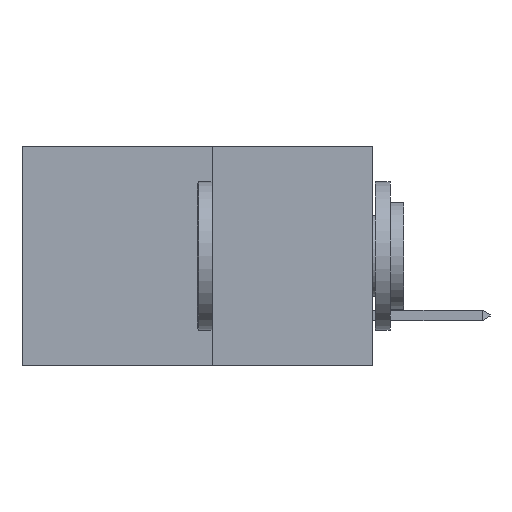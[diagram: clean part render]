
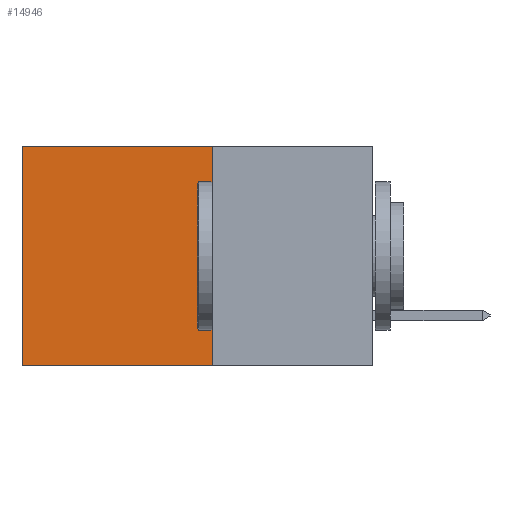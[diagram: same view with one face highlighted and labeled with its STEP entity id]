
A CAD part, left-side view. The second image highlights one B-rep face of the part: STEP entity #14946.
In plain terms, the highlighted planar face has unit normal (-1, 0, 0).
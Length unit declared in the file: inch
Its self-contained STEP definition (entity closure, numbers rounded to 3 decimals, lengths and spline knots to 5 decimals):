
#177 = DIRECTION ( 'NONE',  ( 0., 1., 0. ) ) ;
#680 = EDGE_CURVE ( 'NONE', #9956, #7408, #4182, .T. ) ;
#739 = VECTOR ( 'NONE', #12004, 39.37008 ) ;
#1069 = CARTESIAN_POINT ( 'NONE',  ( 0.277, 0.59, 0. ) ) ;
#1092 = CARTESIAN_POINT ( 'NONE',  ( 0.277, 0.27, -0.37 ) ) ;
#1283 = LINE ( 'NONE', #14451, #11419 ) ;
#1910 = FACE_OUTER_BOUND ( 'NONE', #10931, .T. ) ;
#3737 = DIRECTION ( 'NONE',  ( 1., 0., 0. ) ) ;
#3913 = LINE ( 'NONE', #15211, #10244 ) ;
#4182 = LINE ( 'NONE', #9151, #739 ) ;
#5187 = CARTESIAN_POINT ( 'NONE',  ( 0.277, 0.59, -0.37 ) ) ;
#5775 = DIRECTION ( 'NONE',  ( 0., 0., -1. ) ) ;
#5854 = ORIENTED_EDGE ( 'NONE', *, *, #15078, .T. ) ;
#6277 = ORIENTED_EDGE ( 'NONE', *, *, #680, .T. ) ;
#7129 = VECTOR ( 'NONE', #13907, 39.37008 ) ;
#7408 = VERTEX_POINT ( 'NONE', #1069 ) ;
#7410 = VERTEX_POINT ( 'NONE', #1092 ) ;
#8767 = CARTESIAN_POINT ( 'NONE',  ( 0.277, 0.27, -0.37 ) ) ;
#8828 = EDGE_CURVE ( 'NONE', #9956, #7410, #1283, .T. ) ;
#9020 = CARTESIAN_POINT ( 'NONE',  ( 0.277, 0.27, 0. ) ) ;
#9151 = CARTESIAN_POINT ( 'NONE',  ( 0.277, 0.27, 0. ) ) ;
#9282 = EDGE_CURVE ( 'NONE', #7410, #10109, #3913, .T. ) ;
#9956 = VERTEX_POINT ( 'NONE', #9020 ) ;
#10109 = VERTEX_POINT ( 'NONE', #13074 ) ;
#10244 = VECTOR ( 'NONE', #177, 39.37008 ) ;
#10931 = EDGE_LOOP ( 'NONE', ( #5854, #12510, #15691, #6277 ) ) ;
#11290 = PLANE ( 'NONE',  #11726 ) ;
#11419 = VECTOR ( 'NONE', #5775, 39.37008 ) ;
#11726 = AXIS2_PLACEMENT_3D ( 'NONE', #8767, #3737, #12529 ) ;
#12004 = DIRECTION ( 'NONE',  ( 0., 1., 0. ) ) ;
#12510 = ORIENTED_EDGE ( 'NONE', *, *, #9282, .F. ) ;
#12529 = DIRECTION ( 'NONE',  ( 0., 0., -1. ) ) ;
#13074 = CARTESIAN_POINT ( 'NONE',  ( 0.277, 0.59, -0.37 ) ) ;
#13729 = LINE ( 'NONE', #5187, #7129 ) ;
#13907 = DIRECTION ( 'NONE',  ( 0., 0., -1. ) ) ;
#14451 = CARTESIAN_POINT ( 'NONE',  ( 0.277, 0.27, -0.37 ) ) ;
#14946 = ADVANCED_FACE ( 'NONE', ( #1910 ), #11290, .F. ) ;
#15078 = EDGE_CURVE ( 'NONE', #7408, #10109, #13729, .T. ) ;
#15211 = CARTESIAN_POINT ( 'NONE',  ( 0.277, 0.27, -0.37 ) ) ;
#15691 = ORIENTED_EDGE ( 'NONE', *, *, #8828, .F. ) ;
